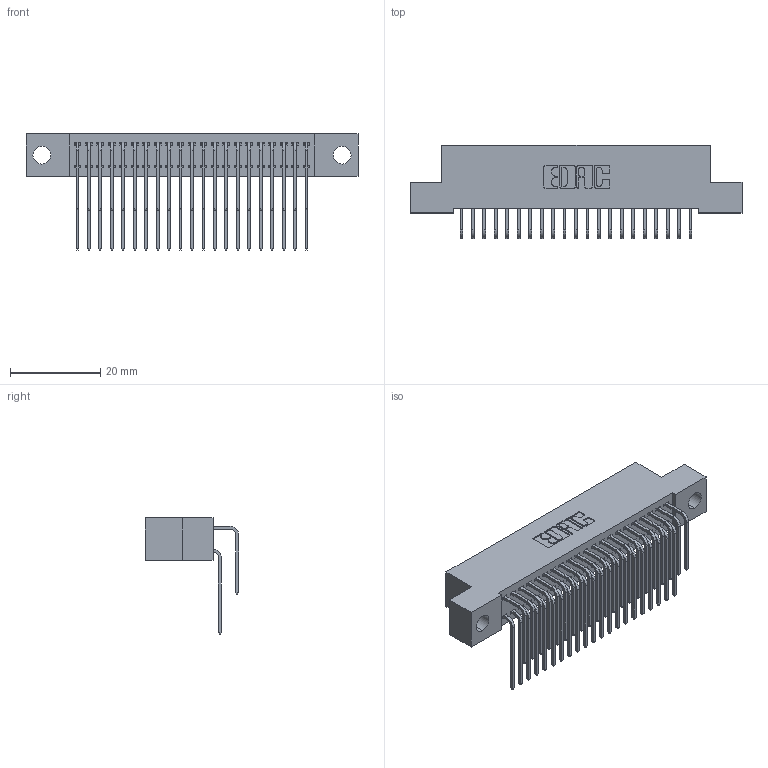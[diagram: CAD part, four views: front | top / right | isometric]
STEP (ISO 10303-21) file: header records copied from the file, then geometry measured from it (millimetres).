
FILE_DESCRIPTION (( 'STEP AP203' ), '1' );
FILE_NAME ('392-042-559-204.STEP', '2018-08-16T14:06:50', ( '' ), ( '' ), 'SwSTEP 2.0', 'SolidWorks 2016', '' );
FILE_SCHEMA (( 'CONFIG_CONTROL_DESIGN' ));
Length unit declared in the file: inch
Products named in the file (4): 342 Part_.156 TH; 345-292-001_558 559 Tail - 1; 345-292-001_559 Tail - 2; 392-042-559-204
Assembly tree (43 placements, depth 2):
  392-042-559-204
    342 Part_.156 TH
    345-292-001_558 559 Tail - 1  x21
    345-292-001_559 Tail - 2  x21
Bounding box: 73.66 x 20.64 x 25.78 mm (x, y, z)
Volume: 6674.2 mm3; surface area: 11266.7 mm2
Topology: 43 solids, 43 shells, 2378 faces, 7061 edges, 4650 vertices
Faces by surface type: plane 1662, cylinder 716
Entity records: 17881 total; most frequent: CARTESIAN_POINT 3037, ORIENTED_EDGE 2922, DIRECTION 2613, EDGE_CURVE 1461, LINE 1293, VECTOR 1293, VERTEX_POINT 970, AXIS2_PLACEMENT_3D 660
